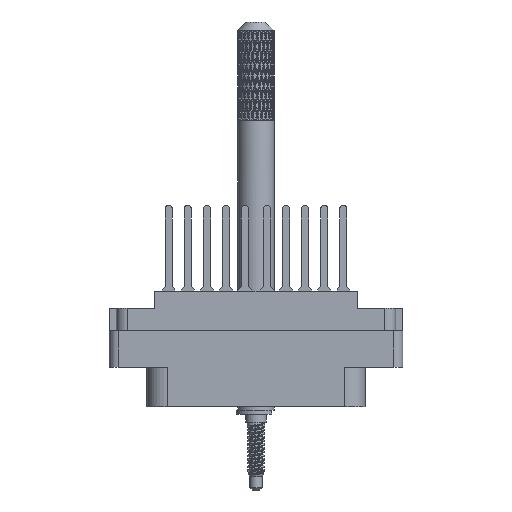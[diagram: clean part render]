
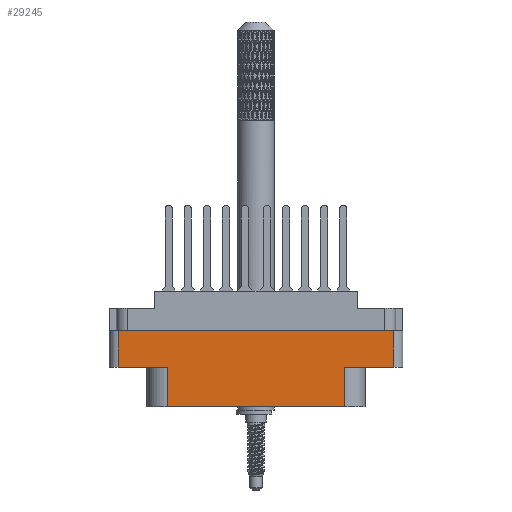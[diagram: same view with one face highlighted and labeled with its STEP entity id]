
A CAD part, front view. The second image highlights one B-rep face of the part: STEP entity #29245.
In plain terms, the highlighted planar face has unit normal (0, -1, 0).
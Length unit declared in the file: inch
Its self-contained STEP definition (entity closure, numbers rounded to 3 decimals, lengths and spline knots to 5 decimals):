
#1776 = LINE ( 'NONE', #87427, #84128 ) ;
#5091 = EDGE_CURVE ( 'NONE', #83013, #82129, #101528, .T. ) ;
#9223 = CARTESIAN_POINT ( 'NONE',  ( 0., -0.438, -0.52 ) ) ;
#11304 = PLANE ( 'NONE',  #97259 ) ;
#11561 = EDGE_CURVE ( 'NONE', #54306, #83013, #68808, .T. ) ;
#11569 = DIRECTION ( 'NONE',  ( 0., 0., 1. ) ) ;
#11956 = LINE ( 'NONE', #22351, #94331 ) ;
#22351 = CARTESIAN_POINT ( 'NONE',  ( -0.604, -0.438, -0.789 ) ) ;
#23583 = DIRECTION ( 'NONE',  ( 0., 0., -1. ) ) ;
#24126 = CARTESIAN_POINT ( 'NONE',  ( 0.938, -0.438, -0.268 ) ) ;
#25224 = DIRECTION ( 'NONE',  ( 1., 0., 0. ) ) ;
#27218 = VECTOR ( 'NONE', #59501, 39.37008 ) ;
#27384 = CARTESIAN_POINT ( 'NONE',  ( 0., -0.438, -0.52 ) ) ;
#29245 = ADVANCED_FACE ( 'NONE', ( #76062 ), #11304, .T. ) ;
#29620 = VERTEX_POINT ( 'NONE', #24126 ) ;
#29715 = VERTEX_POINT ( 'NONE', #64591 ) ;
#30133 = ORIENTED_EDGE ( 'NONE', *, *, #55168, .T. ) ;
#34095 = CARTESIAN_POINT ( 'NONE',  ( -0.604, -0.438, -0.789 ) ) ;
#35943 = CARTESIAN_POINT ( 'NONE',  ( 0.938, -0.438, -0.789 ) ) ;
#36049 = DIRECTION ( 'NONE',  ( 1., 0., 0. ) ) ;
#38381 = DIRECTION ( 'NONE',  ( 0., 0., -1. ) ) ;
#39305 = ORIENTED_EDGE ( 'NONE', *, *, #44770, .T. ) ;
#40318 = EDGE_LOOP ( 'NONE', ( #77834, #95255, #99480, #39305, #97364, #91932, #67152, #30133 ) ) ;
#40548 = CARTESIAN_POINT ( 'NONE',  ( 0.604, -0.438, -0.52 ) ) ;
#41989 = EDGE_CURVE ( 'NONE', #52594, #82129, #100932, .T. ) ;
#42154 = DIRECTION ( 'NONE',  ( 1., 0., 0. ) ) ;
#43035 = CARTESIAN_POINT ( 'NONE',  ( -1., -0.438, -0.789 ) ) ;
#44770 = EDGE_CURVE ( 'NONE', #63303, #54306, #11956, .T. ) ;
#45526 = VERTEX_POINT ( 'NONE', #71301 ) ;
#50031 = VECTOR ( 'NONE', #36049, 39.37008 ) ;
#50685 = DIRECTION ( 'NONE',  ( 0., 0., -1. ) ) ;
#52594 = VERTEX_POINT ( 'NONE', #102585 ) ;
#53544 = LINE ( 'NONE', #9223, #103505 ) ;
#54306 = VERTEX_POINT ( 'NONE', #34095 ) ;
#55168 = EDGE_CURVE ( 'NONE', #52594, #29620, #66267, .T. ) ;
#58741 = DIRECTION ( 'NONE',  ( 0., -1., 0. ) ) ;
#59459 = CARTESIAN_POINT ( 'NONE',  ( -1., -0.438, -0.789 ) ) ;
#59501 = DIRECTION ( 'NONE',  ( -1., 0., 0. ) ) ;
#63303 = VERTEX_POINT ( 'NONE', #97913 ) ;
#64591 = CARTESIAN_POINT ( 'NONE',  ( -0.938, -0.438, -0.268 ) ) ;
#65373 = VECTOR ( 'NONE', #72686, 39.37008 ) ;
#66267 = LINE ( 'NONE', #35943, #76277 ) ;
#67152 = ORIENTED_EDGE ( 'NONE', *, *, #41989, .F. ) ;
#68808 = LINE ( 'NONE', #59459, #50031 ) ;
#71301 = CARTESIAN_POINT ( 'NONE',  ( -0.938, -0.438, -0.52 ) ) ;
#72686 = DIRECTION ( 'NONE',  ( 0., 0., 1. ) ) ;
#73373 = EDGE_CURVE ( 'NONE', #45526, #63303, #53544, .T. ) ;
#73640 = CARTESIAN_POINT ( 'NONE',  ( 0.604, -0.438, -0.52 ) ) ;
#76062 = FACE_OUTER_BOUND ( 'NONE', #40318, .T. ) ;
#76277 = VECTOR ( 'NONE', #11569, 39.37008 ) ;
#77724 = VECTOR ( 'NONE', #42154, 39.37008 ) ;
#77834 = ORIENTED_EDGE ( 'NONE', *, *, #89506, .F. ) ;
#77945 = EDGE_CURVE ( 'NONE', #29715, #45526, #1776, .T. ) ;
#81901 = CARTESIAN_POINT ( 'NONE',  ( 0., -0.438, -0.268 ) ) ;
#82129 = VERTEX_POINT ( 'NONE', #73640 ) ;
#83013 = VERTEX_POINT ( 'NONE', #86590 ) ;
#84128 = VECTOR ( 'NONE', #23583, 39.37008 ) ;
#86590 = CARTESIAN_POINT ( 'NONE',  ( 0.604, -0.438, -0.789 ) ) ;
#87427 = CARTESIAN_POINT ( 'NONE',  ( -0.938, -0.438, -0.789 ) ) ;
#89506 = EDGE_CURVE ( 'NONE', #29715, #29620, #91376, .T. ) ;
#91376 = LINE ( 'NONE', #81901, #77724 ) ;
#91932 = ORIENTED_EDGE ( 'NONE', *, *, #5091, .T. ) ;
#94331 = VECTOR ( 'NONE', #38381, 39.37008 ) ;
#95255 = ORIENTED_EDGE ( 'NONE', *, *, #77945, .T. ) ;
#97259 = AXIS2_PLACEMENT_3D ( 'NONE', #43035, #58741, #50685 ) ;
#97364 = ORIENTED_EDGE ( 'NONE', *, *, #11561, .T. ) ;
#97913 = CARTESIAN_POINT ( 'NONE',  ( -0.604, -0.438, -0.52 ) ) ;
#99480 = ORIENTED_EDGE ( 'NONE', *, *, #73373, .T. ) ;
#100932 = LINE ( 'NONE', #27384, #27218 ) ;
#101528 = LINE ( 'NONE', #40548, #65373 ) ;
#102585 = CARTESIAN_POINT ( 'NONE',  ( 0.938, -0.438, -0.52 ) ) ;
#103505 = VECTOR ( 'NONE', #25224, 39.37008 ) ;
